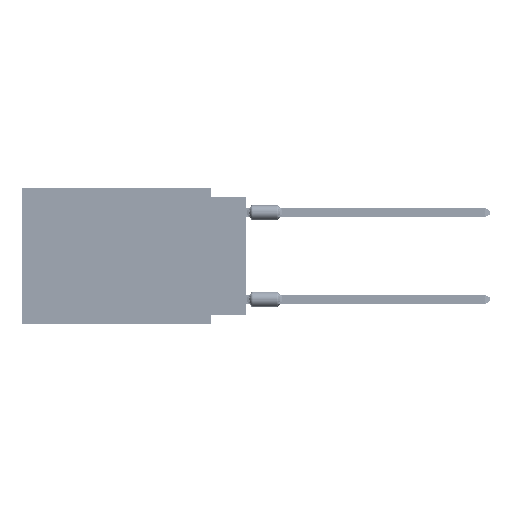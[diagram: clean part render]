
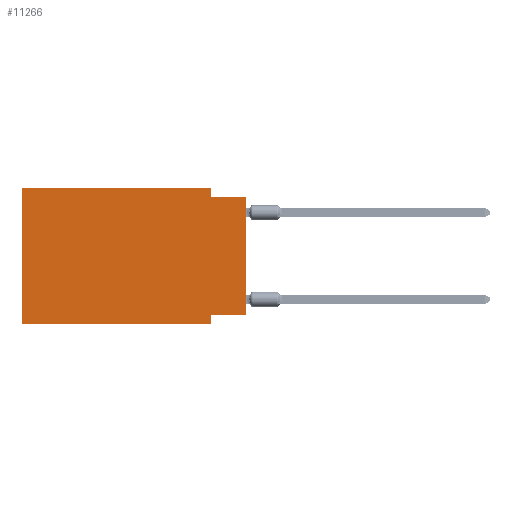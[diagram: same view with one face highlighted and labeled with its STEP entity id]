
A CAD part, left-side view. The second image highlights one B-rep face of the part: STEP entity #11266.
In plain terms, the highlighted planar face has unit normal (-1, 0, 0).
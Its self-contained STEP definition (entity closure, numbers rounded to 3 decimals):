
#658 = VERTEX_POINT ( 'NONE', #20873 ) ;
#3582 = VERTEX_POINT ( 'NONE', #71352 ) ;
#4097 = VERTEX_POINT ( 'NONE', #26986 ) ;
#4589 = EDGE_CURVE ( 'NONE', #658, #73062, #23329, .T. ) ;
#6060 = VECTOR ( 'NONE', #72526, 1000. ) ;
#6591 = VECTOR ( 'NONE', #54371, 1000. ) ;
#7444 = VERTEX_POINT ( 'NONE', #71163 ) ;
#7594 = AXIS2_PLACEMENT_3D ( 'NONE', #75417, #63098, #16181 ) ;
#8183 = VECTOR ( 'NONE', #58304, 1000. ) ;
#9182 = LINE ( 'NONE', #14568, #11934 ) ;
#9295 = FACE_OUTER_BOUND ( 'NONE', #70417, .T. ) ;
#9603 = EDGE_CURVE ( 'NONE', #54109, #4097, #60573, .T. ) ;
#9605 = CARTESIAN_POINT ( 'NONE',  ( 0., 0., -9.271 ) ) ;
#11266 = ADVANCED_FACE ( 'NONE', ( #9295 ), #15051, .F. ) ;
#11934 = VECTOR ( 'NONE', #32255, 1000. ) ;
#12016 = VERTEX_POINT ( 'NONE', #37965 ) ;
#13165 = ORIENTED_EDGE ( 'NONE', *, *, #47786, .F. ) ;
#14568 = CARTESIAN_POINT ( 'NONE',  ( 0., 2.54, -9.906 ) ) ;
#15051 = PLANE ( 'NONE',  #7594 ) ;
#16181 = DIRECTION ( 'NONE',  ( 0., 0., -1. ) ) ;
#16875 = ORIENTED_EDGE ( 'NONE', *, *, #4589, .T. ) ;
#18623 = CARTESIAN_POINT ( 'NONE',  ( 0., 16.383, 0. ) ) ;
#20392 = DIRECTION ( 'NONE',  ( 0., 1., 0. ) ) ;
#20873 = CARTESIAN_POINT ( 'NONE',  ( 0., 16.383, -9.906 ) ) ;
#23329 = LINE ( 'NONE', #47908, #8183 ) ;
#23424 = ORIENTED_EDGE ( 'NONE', *, *, #9603, .F. ) ;
#24761 = LINE ( 'NONE', #18623, #6591 ) ;
#26599 = LINE ( 'NONE', #43909, #69675 ) ;
#26979 = EDGE_CURVE ( 'NONE', #12016, #73062, #9182, .T. ) ;
#26986 = CARTESIAN_POINT ( 'NONE',  ( 0., 2.54, -0.635 ) ) ;
#31740 = CARTESIAN_POINT ( 'NONE',  ( 0., 2.54, 0. ) ) ;
#32255 = DIRECTION ( 'NONE',  ( 0., 0., -1. ) ) ;
#32523 = CARTESIAN_POINT ( 'NONE',  ( 0., 0., -0.635 ) ) ;
#33224 = ORIENTED_EDGE ( 'NONE', *, *, #69826, .T. ) ;
#33281 = DIRECTION ( 'NONE',  ( 0., -1., 0. ) ) ;
#35141 = VECTOR ( 'NONE', #20392, 1000. ) ;
#37006 = ORIENTED_EDGE ( 'NONE', *, *, #57103, .F. ) ;
#37965 = CARTESIAN_POINT ( 'NONE',  ( 0., 2.54, -9.271 ) ) ;
#37974 = VERTEX_POINT ( 'NONE', #67232 ) ;
#42147 = DIRECTION ( 'NONE',  ( 0., 0., -1. ) ) ;
#42778 = DIRECTION ( 'NONE',  ( 0., 0., 1. ) ) ;
#43909 = CARTESIAN_POINT ( 'NONE',  ( 0., 0., 0. ) ) ;
#44045 = LINE ( 'NONE', #32523, #6060 ) ;
#47786 = EDGE_CURVE ( 'NONE', #7444, #12016, #62275, .T. ) ;
#47908 = CARTESIAN_POINT ( 'NONE',  ( 0., 16.383, -9.906 ) ) ;
#51651 = CARTESIAN_POINT ( 'NONE',  ( 0., 2.54, 0. ) ) ;
#54109 = VERTEX_POINT ( 'NONE', #51651 ) ;
#54371 = DIRECTION ( 'NONE',  ( 0., 0., 1. ) ) ;
#56367 = ORIENTED_EDGE ( 'NONE', *, *, #63857, .F. ) ;
#56558 = VECTOR ( 'NONE', #42147, 1000. ) ;
#57103 = EDGE_CURVE ( 'NONE', #4097, #37974, #44045, .T. ) ;
#57846 = LINE ( 'NONE', #75187, #68501 ) ;
#58304 = DIRECTION ( 'NONE',  ( 0., -1., 0. ) ) ;
#60573 = LINE ( 'NONE', #31740, #56558 ) ;
#61732 = ORIENTED_EDGE ( 'NONE', *, *, #26979, .F. ) ;
#62275 = LINE ( 'NONE', #9605, #35141 ) ;
#63098 = DIRECTION ( 'NONE',  ( 1., 0., 0. ) ) ;
#63857 = EDGE_CURVE ( 'NONE', #658, #3582, #24761, .T. ) ;
#67232 = CARTESIAN_POINT ( 'NONE',  ( 0., 0., -0.635 ) ) ;
#68423 = CARTESIAN_POINT ( 'NONE',  ( 0., 2.54, -9.906 ) ) ;
#68501 = VECTOR ( 'NONE', #33281, 1000. ) ;
#69675 = VECTOR ( 'NONE', #42778, 1000. ) ;
#69826 = EDGE_CURVE ( 'NONE', #7444, #37974, #26599, .T. ) ;
#70417 = EDGE_LOOP ( 'NONE', ( #33224, #37006, #23424, #71655, #56367, #16875, #61732, #13165 ) ) ;
#71163 = CARTESIAN_POINT ( 'NONE',  ( 0., 0., -9.271 ) ) ;
#71352 = CARTESIAN_POINT ( 'NONE',  ( 0., 16.383, 0. ) ) ;
#71655 = ORIENTED_EDGE ( 'NONE', *, *, #75163, .F. ) ;
#72526 = DIRECTION ( 'NONE',  ( 0., -1., 0. ) ) ;
#73062 = VERTEX_POINT ( 'NONE', #68423 ) ;
#75163 = EDGE_CURVE ( 'NONE', #3582, #54109, #57846, .T. ) ;
#75187 = CARTESIAN_POINT ( 'NONE',  ( 0., 16.383, 0. ) ) ;
#75417 = CARTESIAN_POINT ( 'NONE',  ( 0., 16.383, 0. ) ) ;
